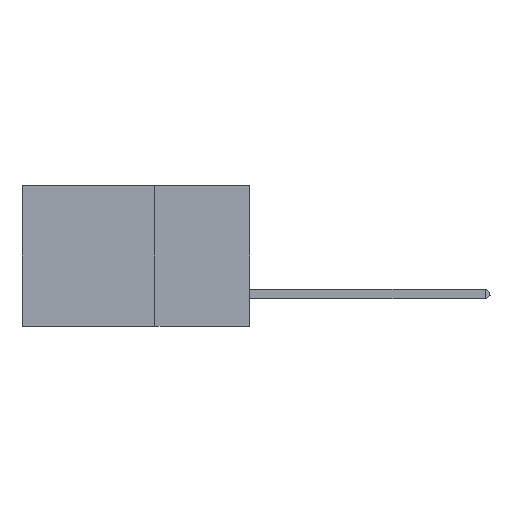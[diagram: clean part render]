
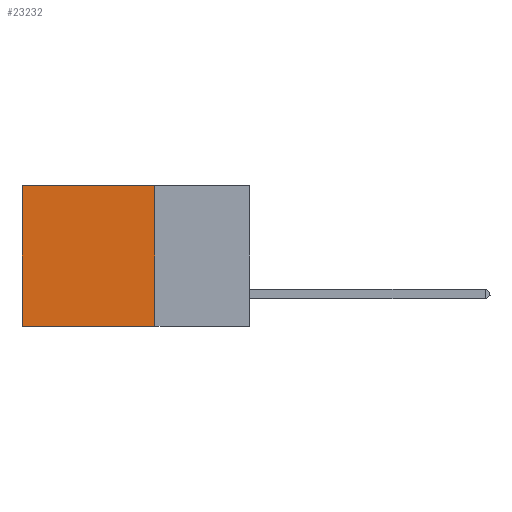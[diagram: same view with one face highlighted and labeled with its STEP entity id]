
A CAD part, left-side view. The second image highlights one B-rep face of the part: STEP entity #23232.
In plain terms, the highlighted planar face has unit normal (-1, 0, 0).
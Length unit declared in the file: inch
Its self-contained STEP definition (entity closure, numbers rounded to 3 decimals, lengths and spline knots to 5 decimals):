
#5853 = DIRECTION ( 'NONE',  ( 0., 1., 0. ) ) ;
#6794 = ORIENTED_EDGE ( 'NONE', *, *, #39349, .T. ) ;
#7653 = CARTESIAN_POINT ( 'NONE',  ( 0.2875, 0.25, -0.37 ) ) ;
#7816 = AXIS2_PLACEMENT_3D ( 'NONE', #13315, #13450, #35583 ) ;
#7847 = VECTOR ( 'NONE', #35661, 39.37008 ) ;
#8991 = VECTOR ( 'NONE', #5853, 39.37008 ) ;
#10512 = EDGE_CURVE ( 'NONE', #24089, #25670, #37132, .T. ) ;
#10756 = LINE ( 'NONE', #26077, #7847 ) ;
#11237 = VERTEX_POINT ( 'NONE', #18488 ) ;
#11407 = CARTESIAN_POINT ( 'NONE',  ( 0.2875, 0.25, 0. ) ) ;
#12469 = CARTESIAN_POINT ( 'NONE',  ( 0.2875, 0.25, 0. ) ) ;
#12842 = EDGE_LOOP ( 'NONE', ( #16000, #14193, #36797, #6794 ) ) ;
#13315 = CARTESIAN_POINT ( 'NONE',  ( 0.2875, 0.25, 0. ) ) ;
#13450 = DIRECTION ( 'NONE',  ( 1., 0., 0. ) ) ;
#13675 = DIRECTION ( 'NONE',  ( 0., 0., -1. ) ) ;
#14193 = ORIENTED_EDGE ( 'NONE', *, *, #37424, .F. ) ;
#14533 = DIRECTION ( 'NONE',  ( 0., 0., -1. ) ) ;
#16000 = ORIENTED_EDGE ( 'NONE', *, *, #10512, .T. ) ;
#16249 = LINE ( 'NONE', #12469, #8991 ) ;
#17244 = CARTESIAN_POINT ( 'NONE',  ( 0.2875, 0.6, 0. ) ) ;
#18035 = FACE_OUTER_BOUND ( 'NONE', #12842, .T. ) ;
#18488 = CARTESIAN_POINT ( 'NONE',  ( 0.2875, 0.25, 0. ) ) ;
#20228 = EDGE_CURVE ( 'NONE', #11237, #26353, #22641, .T. ) ;
#22641 = LINE ( 'NONE', #11407, #32928 ) ;
#23232 = ADVANCED_FACE ( 'NONE', ( #18035 ), #25875, .F. ) ;
#24089 = VERTEX_POINT ( 'NONE', #31557 ) ;
#25670 = VERTEX_POINT ( 'NONE', #34033 ) ;
#25875 = PLANE ( 'NONE',  #7816 ) ;
#26077 = CARTESIAN_POINT ( 'NONE',  ( 0.2875, 0.25, -0.37 ) ) ;
#26353 = VERTEX_POINT ( 'NONE', #7653 ) ;
#28886 = VECTOR ( 'NONE', #13675, 39.37008 ) ;
#31557 = CARTESIAN_POINT ( 'NONE',  ( 0.2875, 0.6, 0. ) ) ;
#32928 = VECTOR ( 'NONE', #14533, 39.37008 ) ;
#34033 = CARTESIAN_POINT ( 'NONE',  ( 0.2875, 0.6, -0.37 ) ) ;
#35583 = DIRECTION ( 'NONE',  ( 0., 0., -1. ) ) ;
#35661 = DIRECTION ( 'NONE',  ( 0., 1., 0. ) ) ;
#36797 = ORIENTED_EDGE ( 'NONE', *, *, #20228, .F. ) ;
#37132 = LINE ( 'NONE', #17244, #28886 ) ;
#37424 = EDGE_CURVE ( 'NONE', #26353, #25670, #10756, .T. ) ;
#39349 = EDGE_CURVE ( 'NONE', #11237, #24089, #16249, .T. ) ;
